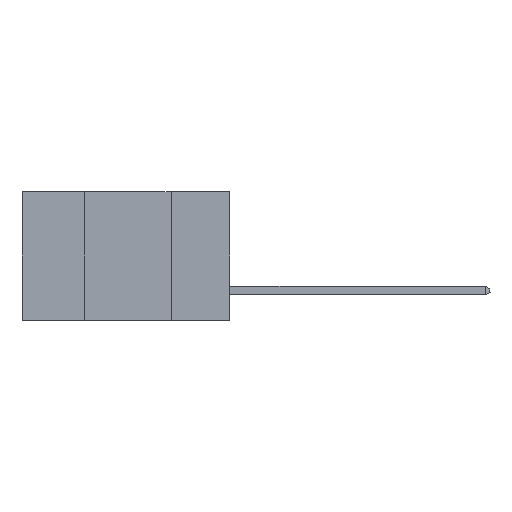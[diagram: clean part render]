
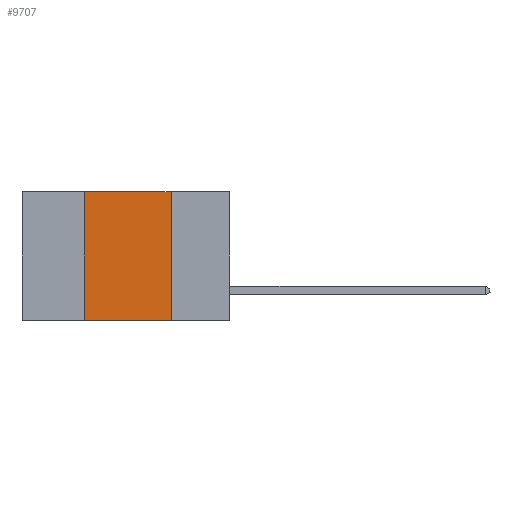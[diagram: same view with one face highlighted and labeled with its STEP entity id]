
A CAD part, left-side view. The second image highlights one B-rep face of the part: STEP entity #9707.
In plain terms, the highlighted planar face has unit normal (-1, 0, 0).
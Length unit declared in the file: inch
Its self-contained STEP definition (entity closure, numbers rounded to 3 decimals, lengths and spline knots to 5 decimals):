
#31 = ORIENTED_EDGE ( 'NONE', *, *, #3458, .T. ) ;
#772 = CARTESIAN_POINT ( 'NONE',  ( 0., 0.6, 0. ) ) ;
#1203 = EDGE_LOOP ( 'NONE', ( #2120, #8834, #3732, #31 ) ) ;
#1258 = DIRECTION ( 'NONE',  ( 0., 0., -1. ) ) ;
#1437 = CARTESIAN_POINT ( 'NONE',  ( 0., 0.42, -0.37 ) ) ;
#1533 = DIRECTION ( 'NONE',  ( 0., 0., -1. ) ) ;
#1627 = AXIS2_PLACEMENT_3D ( 'NONE', #772, #5450, #1533 ) ;
#1803 = VECTOR ( 'NONE', #9895, 39.37008 ) ;
#2120 = ORIENTED_EDGE ( 'NONE', *, *, #5418, .F. ) ;
#2152 = VERTEX_POINT ( 'NONE', #5879 ) ;
#2294 = VERTEX_POINT ( 'NONE', #4534 ) ;
#2314 = FACE_OUTER_BOUND ( 'NONE', #1203, .T. ) ;
#2730 = CARTESIAN_POINT ( 'NONE',  ( 0., 0.6, 0. ) ) ;
#2779 = EDGE_CURVE ( 'NONE', #6917, #2152, #5506, .T. ) ;
#3458 = EDGE_CURVE ( 'NONE', #6917, #5449, #3997, .T. ) ;
#3523 = EDGE_CURVE ( 'NONE', #2152, #2294, #4103, .T. ) ;
#3732 = ORIENTED_EDGE ( 'NONE', *, *, #2779, .F. ) ;
#3756 = CARTESIAN_POINT ( 'NONE',  ( 0., 0.17, 0. ) ) ;
#3997 = LINE ( 'NONE', #9674, #6198 ) ;
#4006 = VECTOR ( 'NONE', #6931, 39.37008 ) ;
#4103 = LINE ( 'NONE', #2730, #1803 ) ;
#4534 = CARTESIAN_POINT ( 'NONE',  ( 0., 0.17, 0. ) ) ;
#5344 = CARTESIAN_POINT ( 'NONE',  ( 0., 0.42, 0. ) ) ;
#5418 = EDGE_CURVE ( 'NONE', #2294, #5449, #8905, .T. ) ;
#5449 = VERTEX_POINT ( 'NONE', #7614 ) ;
#5450 = DIRECTION ( 'NONE',  ( 1., 0., 0. ) ) ;
#5506 = LINE ( 'NONE', #5344, #4006 ) ;
#5879 = CARTESIAN_POINT ( 'NONE',  ( 0., 0.42, 0. ) ) ;
#6198 = VECTOR ( 'NONE', #6404, 39.37008 ) ;
#6404 = DIRECTION ( 'NONE',  ( 0., -1., 0. ) ) ;
#6917 = VERTEX_POINT ( 'NONE', #1437 ) ;
#6931 = DIRECTION ( 'NONE',  ( 0., 0., 1. ) ) ;
#7614 = CARTESIAN_POINT ( 'NONE',  ( 0., 0.17, -0.37 ) ) ;
#7620 = VECTOR ( 'NONE', #1258, 39.37008 ) ;
#8834 = ORIENTED_EDGE ( 'NONE', *, *, #3523, .F. ) ;
#8905 = LINE ( 'NONE', #3756, #7620 ) ;
#9523 = PLANE ( 'NONE',  #1627 ) ;
#9674 = CARTESIAN_POINT ( 'NONE',  ( 0., 0.6, -0.37 ) ) ;
#9707 = ADVANCED_FACE ( 'NONE', ( #2314 ), #9523, .F. ) ;
#9895 = DIRECTION ( 'NONE',  ( 0., -1., 0. ) ) ;
